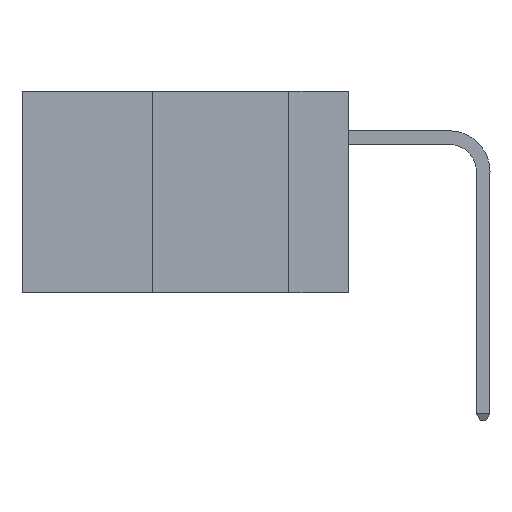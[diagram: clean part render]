
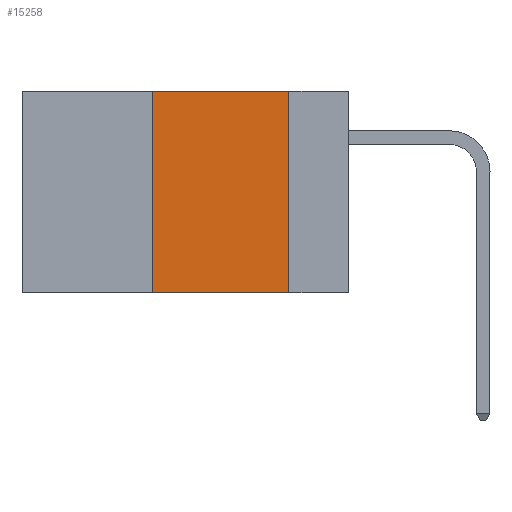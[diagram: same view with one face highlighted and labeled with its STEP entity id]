
A CAD part, left-side view. The second image highlights one B-rep face of the part: STEP entity #15258.
In plain terms, the highlighted planar face has unit normal (-1, 0, 0).
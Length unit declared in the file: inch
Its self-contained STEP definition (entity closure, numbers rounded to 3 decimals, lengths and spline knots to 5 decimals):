
#521 = LINE ( 'NONE', #12348, #4991 ) ;
#670 = EDGE_CURVE ( 'NONE', #12155, #5403, #9041, .T. ) ;
#1033 = CARTESIAN_POINT ( 'NONE',  ( 0., 0.36, 0. ) ) ;
#1302 = ORIENTED_EDGE ( 'NONE', *, *, #9427, .T. ) ;
#1532 = CARTESIAN_POINT ( 'NONE',  ( 0., 0.6, 0. ) ) ;
#2133 = VECTOR ( 'NONE', #6908, 39.37008 ) ;
#4140 = EDGE_LOOP ( 'NONE', ( #15942, #15868, #6048, #1302 ) ) ;
#4991 = VECTOR ( 'NONE', #16335, 39.37008 ) ;
#5403 = VERTEX_POINT ( 'NONE', #7109 ) ;
#5783 = PLANE ( 'NONE',  #14001 ) ;
#5889 = VERTEX_POINT ( 'NONE', #9526 ) ;
#5942 = CARTESIAN_POINT ( 'NONE',  ( 0., 0.11, 0. ) ) ;
#6048 = ORIENTED_EDGE ( 'NONE', *, *, #11187, .F. ) ;
#6176 = VECTOR ( 'NONE', #11244, 39.37008 ) ;
#6908 = DIRECTION ( 'NONE',  ( 0., 0., 1. ) ) ;
#6910 = FACE_OUTER_BOUND ( 'NONE', #4140, .T. ) ;
#6927 = CARTESIAN_POINT ( 'NONE',  ( 0., 0.11, 0. ) ) ;
#7109 = CARTESIAN_POINT ( 'NONE',  ( 0., 0.11, -0.37 ) ) ;
#9041 = LINE ( 'NONE', #5942, #17583 ) ;
#9427 = EDGE_CURVE ( 'NONE', #5889, #5403, #14491, .T. ) ;
#9526 = CARTESIAN_POINT ( 'NONE',  ( 0., 0.36, -0.37 ) ) ;
#11187 = EDGE_CURVE ( 'NONE', #5889, #13619, #12776, .T. ) ;
#11244 = DIRECTION ( 'NONE',  ( 0., -1., 0. ) ) ;
#11296 = CARTESIAN_POINT ( 'NONE',  ( 0., 0.6, -0.37 ) ) ;
#12155 = VERTEX_POINT ( 'NONE', #6927 ) ;
#12348 = CARTESIAN_POINT ( 'NONE',  ( 0., 0.6, 0. ) ) ;
#12776 = LINE ( 'NONE', #13656, #2133 ) ;
#13619 = VERTEX_POINT ( 'NONE', #1033 ) ;
#13656 = CARTESIAN_POINT ( 'NONE',  ( 0., 0.36, 0. ) ) ;
#14001 = AXIS2_PLACEMENT_3D ( 'NONE', #1532, #15817, #15150 ) ;
#14210 = DIRECTION ( 'NONE',  ( 0., 0., -1. ) ) ;
#14491 = LINE ( 'NONE', #11296, #6176 ) ;
#15150 = DIRECTION ( 'NONE',  ( 0., 0., -1. ) ) ;
#15258 = ADVANCED_FACE ( 'NONE', ( #6910 ), #5783, .F. ) ;
#15817 = DIRECTION ( 'NONE',  ( 1., 0., 0. ) ) ;
#15849 = EDGE_CURVE ( 'NONE', #13619, #12155, #521, .T. ) ;
#15868 = ORIENTED_EDGE ( 'NONE', *, *, #15849, .F. ) ;
#15942 = ORIENTED_EDGE ( 'NONE', *, *, #670, .F. ) ;
#16335 = DIRECTION ( 'NONE',  ( 0., -1., 0. ) ) ;
#17583 = VECTOR ( 'NONE', #14210, 39.37008 ) ;
